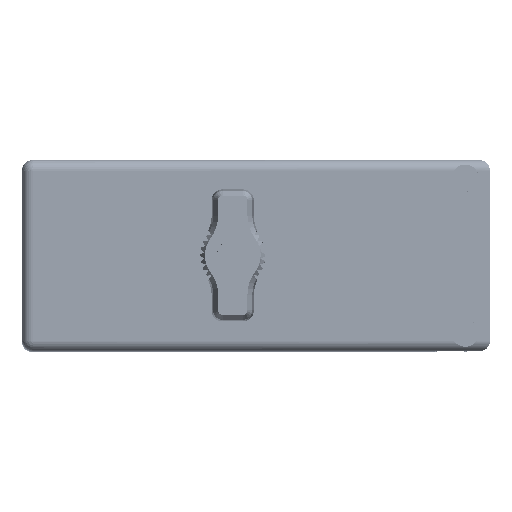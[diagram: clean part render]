
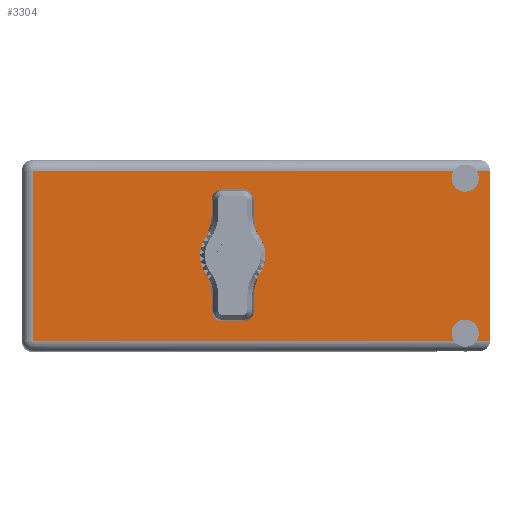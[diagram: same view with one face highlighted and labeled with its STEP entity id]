
A CAD part, top view. The second image highlights one B-rep face of the part: STEP entity #3304.
In plain terms, the highlighted face is planar.
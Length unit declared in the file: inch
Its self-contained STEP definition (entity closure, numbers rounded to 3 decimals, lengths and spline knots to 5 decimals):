
#264 = CIRCLE ( 'NONE', #29194, 0.125 ) ;
#358 = CARTESIAN_POINT ( 'NONE',  ( 1.57281, 1.675, 0.547 ) ) ;
#1883 = ORIENTED_EDGE ( 'NONE', *, *, #23837, .T. ) ;
#3304 = ADVANCED_FACE ( 'NONE', ( #81611, #61806 ), #60358, .T. ) ;
#3413 = DIRECTION ( 'NONE',  ( 0., 0., 1. ) ) ;
#4209 = CARTESIAN_POINT ( 'NONE',  ( 1.499, 1.675, 0.4125 ) ) ;
#4683 = DIRECTION ( 'NONE',  ( -1., 0., 0. ) ) ;
#6624 = CARTESIAN_POINT ( 'NONE',  ( -1.289, 1.675, -0.617 ) ) ;
#6926 = VERTEX_POINT ( 'NONE', #26903 ) ;
#8466 = VERTEX_POINT ( 'NONE', #62322 ) ;
#9006 = CIRCLE ( 'NONE', #83258, 0.125 ) ;
#9915 = VECTOR ( 'NONE', #50572, 39.37008 ) ;
#10372 = EDGE_LOOP ( 'NONE', ( #56472, #41699 ) ) ;
#11654 = AXIS2_PLACEMENT_3D ( 'NONE', #39259, #38665, #26121 ) ;
#12421 = AXIS2_PLACEMENT_3D ( 'NONE', #23589, #76770, #49967 ) ;
#12948 = CARTESIAN_POINT ( 'NONE',  ( -1.359, 1.675, -0.617 ) ) ;
#14196 = DIRECTION ( 'NONE',  ( 0., 0., 1. ) ) ;
#14808 = DIRECTION ( 'NONE',  ( -1., 0., 0. ) ) ;
#17160 = VECTOR ( 'NONE', #4683, 39.37008 ) ;
#17346 = CARTESIAN_POINT ( 'NONE',  ( 1.42519, 1.675, 0.547 ) ) ;
#17459 = VERTEX_POINT ( 'NONE', #4209 ) ;
#17522 = CARTESIAN_POINT ( 'NONE',  ( -1.359, 1.675, -0.547 ) ) ;
#18986 = ORIENTED_EDGE ( 'NONE', *, *, #62487, .T. ) ;
#21032 = ORIENTED_EDGE ( 'NONE', *, *, #78808, .F. ) ;
#21739 = AXIS2_PLACEMENT_3D ( 'NONE', #60205, #40044, #26042 ) ;
#22326 = DIRECTION ( 'NONE',  ( 0., 1., 0. ) ) ;
#22393 = CIRCLE ( 'NONE', #81539, 0.0875 ) ;
#22694 = EDGE_CURVE ( 'NONE', #74211, #44934, #9006, .T. ) ;
#23589 = CARTESIAN_POINT ( 'NONE',  ( 1.499, 1.675, 0.5 ) ) ;
#23837 = EDGE_CURVE ( 'NONE', #82738, #69124, #84104, .T. ) ;
#25037 = EDGE_CURVE ( 'NONE', #44934, #74211, #264, .T. ) ;
#25311 = EDGE_CURVE ( 'NONE', #63691, #8466, #25406, .T. ) ;
#25406 = LINE ( 'NONE', #36793, #44176 ) ;
#26042 = DIRECTION ( 'NONE',  ( 0., 0., 1. ) ) ;
#26121 = DIRECTION ( 'NONE',  ( 0., 0., 1. ) ) ;
#26903 = CARTESIAN_POINT ( 'NONE',  ( -1.289, 1.675, 0.547 ) ) ;
#27811 = LINE ( 'NONE', #77077, #9915 ) ;
#28535 = DIRECTION ( 'NONE',  ( 0., 0., 1. ) ) ;
#29194 = AXIS2_PLACEMENT_3D ( 'NONE', #41165, #54341, #14196 ) ;
#30985 = ORIENTED_EDGE ( 'NONE', *, *, #25311, .F. ) ;
#31647 = DIRECTION ( 'NONE',  ( 0., 0., 1. ) ) ;
#31978 = EDGE_CURVE ( 'NONE', #74364, #8466, #27811, .T. ) ;
#32282 = VERTEX_POINT ( 'NONE', #80740 ) ;
#32857 = CIRCLE ( 'NONE', #11654, 0.0875 ) ;
#33200 = DIRECTION ( 'NONE',  ( -1., 0., 0. ) ) ;
#33845 = CIRCLE ( 'NONE', #21739, 0.0875 ) ;
#33973 = ORIENTED_EDGE ( 'NONE', *, *, #54599, .F. ) ;
#34374 = VECTOR ( 'NONE', #14808, 39.37008 ) ;
#35472 = EDGE_LOOP ( 'NONE', ( #18986, #33973, #71874, #84299, #30985, #41926, #80127, #21032, #1883, #55250 ) ) ;
#36793 = CARTESIAN_POINT ( 'NONE',  ( 1.659, 1.675, 0.617 ) ) ;
#38665 = DIRECTION ( 'NONE',  ( 0., 1., 0. ) ) ;
#38777 = CARTESIAN_POINT ( 'NONE',  ( -1.289, 1.675, -0.547 ) ) ;
#39230 = VERTEX_POINT ( 'NONE', #17346 ) ;
#39259 = CARTESIAN_POINT ( 'NONE',  ( 1.499, 1.675, -0.5 ) ) ;
#40044 = DIRECTION ( 'NONE',  ( 0., 1., 0. ) ) ;
#40678 = LINE ( 'NONE', #67482, #34374 ) ;
#41165 = CARTESIAN_POINT ( 'NONE',  ( 0., 1.675, 0. ) ) ;
#41699 = ORIENTED_EDGE ( 'NONE', *, *, #25037, .F. ) ;
#41926 = ORIENTED_EDGE ( 'NONE', *, *, #82970, .T. ) ;
#44176 = VECTOR ( 'NONE', #3413, 39.37008 ) ;
#44190 = DIRECTION ( 'NONE',  ( 0., 1., 0. ) ) ;
#44833 = VECTOR ( 'NONE', #79696, 39.37008 ) ;
#44934 = VERTEX_POINT ( 'NONE', #71633 ) ;
#45077 = CARTESIAN_POINT ( 'NONE',  ( 0., 1.675, 0. ) ) ;
#45205 = CARTESIAN_POINT ( 'NONE',  ( 1.499, 1.675, -0.4125 ) ) ;
#49008 = CARTESIAN_POINT ( 'NONE',  ( 1.499, 1.675, -0.5 ) ) ;
#49967 = DIRECTION ( 'NONE',  ( 0., 0., 1. ) ) ;
#50572 = DIRECTION ( 'NONE',  ( 1., 0., 0. ) ) ;
#51235 = CARTESIAN_POINT ( 'NONE',  ( 1.42519, 1.675, -0.547 ) ) ;
#51963 = CIRCLE ( 'NONE', #12421, 0.0875 ) ;
#53223 = EDGE_CURVE ( 'NONE', #69124, #6926, #76127, .T. ) ;
#54341 = DIRECTION ( 'NONE',  ( 0., 1., 0. ) ) ;
#54599 = EDGE_CURVE ( 'NONE', #17459, #39230, #51963, .T. ) ;
#55250 = ORIENTED_EDGE ( 'NONE', *, *, #53223, .T. ) ;
#56472 = ORIENTED_EDGE ( 'NONE', *, *, #22694, .F. ) ;
#57236 = CARTESIAN_POINT ( 'NONE',  ( 1.659, 1.675, 0.547 ) ) ;
#59402 = AXIS2_PLACEMENT_3D ( 'NONE', #12948, #72588, #33200 ) ;
#60205 = CARTESIAN_POINT ( 'NONE',  ( 1.499, 1.675, 0.5 ) ) ;
#60271 = EDGE_CURVE ( 'NONE', #75062, #32282, #32857, .T. ) ;
#60358 = PLANE ( 'NONE',  #59402 ) ;
#61487 = EDGE_CURVE ( 'NONE', #74364, #17459, #33845, .T. ) ;
#61806 = FACE_OUTER_BOUND ( 'NONE', #35472, .T. ) ;
#62322 = CARTESIAN_POINT ( 'NONE',  ( 1.659, 1.675, 0.547 ) ) ;
#62487 = EDGE_CURVE ( 'NONE', #6926, #39230, #84852, .T. ) ;
#63691 = VERTEX_POINT ( 'NONE', #78665 ) ;
#66730 = CARTESIAN_POINT ( 'NONE',  ( 0., 1.675, 0.125 ) ) ;
#67079 = VECTOR ( 'NONE', #77033, 39.37008 ) ;
#67482 = CARTESIAN_POINT ( 'NONE',  ( -1.359, 1.675, -0.547 ) ) ;
#69124 = VERTEX_POINT ( 'NONE', #38777 ) ;
#71633 = CARTESIAN_POINT ( 'NONE',  ( 0., 1.675, -0.125 ) ) ;
#71874 = ORIENTED_EDGE ( 'NONE', *, *, #61487, .F. ) ;
#72588 = DIRECTION ( 'NONE',  ( 0., 1., 0. ) ) ;
#74211 = VERTEX_POINT ( 'NONE', #66730 ) ;
#74364 = VERTEX_POINT ( 'NONE', #358 ) ;
#75062 = VERTEX_POINT ( 'NONE', #45205 ) ;
#76127 = LINE ( 'NONE', #6624, #44833 ) ;
#76770 = DIRECTION ( 'NONE',  ( 0., 1., 0. ) ) ;
#77033 = DIRECTION ( 'NONE',  ( 1., 0., 0. ) ) ;
#77077 = CARTESIAN_POINT ( 'NONE',  ( 1.659, 1.675, 0.547 ) ) ;
#78665 = CARTESIAN_POINT ( 'NONE',  ( 1.659, 1.675, -0.547 ) ) ;
#78808 = EDGE_CURVE ( 'NONE', #82738, #75062, #22393, .T. ) ;
#79696 = DIRECTION ( 'NONE',  ( 0., 0., 1. ) ) ;
#80127 = ORIENTED_EDGE ( 'NONE', *, *, #60271, .F. ) ;
#80740 = CARTESIAN_POINT ( 'NONE',  ( 1.57281, 1.675, -0.547 ) ) ;
#81539 = AXIS2_PLACEMENT_3D ( 'NONE', #49008, #22326, #28535 ) ;
#81611 = FACE_BOUND ( 'NONE', #10372, .T. ) ;
#82738 = VERTEX_POINT ( 'NONE', #51235 ) ;
#82970 = EDGE_CURVE ( 'NONE', #63691, #32282, #40678, .T. ) ;
#83258 = AXIS2_PLACEMENT_3D ( 'NONE', #45077, #44190, #31647 ) ;
#84104 = LINE ( 'NONE', #17522, #17160 ) ;
#84299 = ORIENTED_EDGE ( 'NONE', *, *, #31978, .T. ) ;
#84852 = LINE ( 'NONE', #57236, #67079 ) ;
